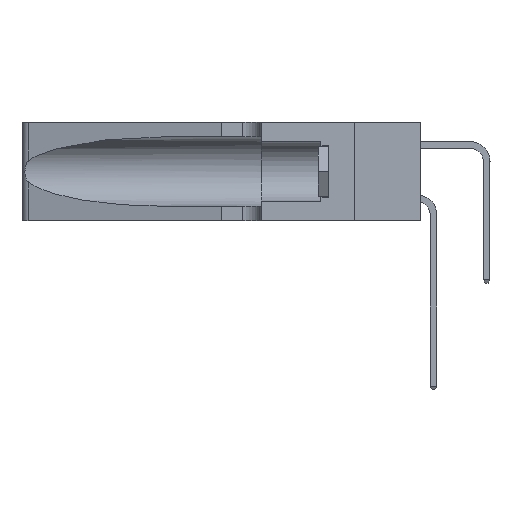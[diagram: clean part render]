
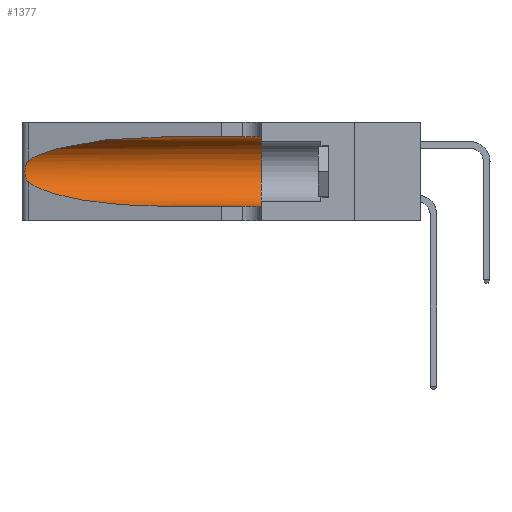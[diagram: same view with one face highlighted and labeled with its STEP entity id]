
A CAD part, left-side view. The second image highlights one B-rep face of the part: STEP entity #1377.
In plain terms, the highlighted cylindrical face has radius 3.308 mm (diameter 6.617 mm), a partial arc.
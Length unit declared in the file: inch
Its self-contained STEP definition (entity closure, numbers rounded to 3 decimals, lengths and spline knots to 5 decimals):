
#92 = ORIENTED_EDGE ( 'NONE', *, *, #10928, .T. ) ;
#417 = CARTESIAN_POINT ( 'NONE',  ( 0.25487, 1.22718, 0.22369 ) ) ;
#531 = CARTESIAN_POINT ( 'NONE',  ( 0.26075, 1.23896, 0.19203 ) ) ;
#1377 = ADVANCED_FACE ( 'NONE', ( #13644 ), #3526, .F. ) ;
#1421 = CARTESIAN_POINT ( 'NONE',  ( 0.1305, 0.72297, 0.05475 ) ) ;
#1494 = CARTESIAN_POINT ( 'NONE',  ( 0.25487, 1.22718, 0.14631 ) ) ;
#2521 = CARTESIAN_POINT ( 'NONE',  ( 0.26017, 1.23833, 0.17102 ) ) ;
#2906 = CARTESIAN_POINT ( 'NONE',  ( 0.1305, 0.35, 0.185 ) ) ;
#3502 = EDGE_CURVE ( 'NONE', #3673, #6131, #13828, .T. ) ;
#3526 = CYLINDRICAL_SURFACE ( 'NONE', #10680, 0.13025 ) ;
#3673 = VERTEX_POINT ( 'NONE', #20260 ) ;
#4228 = VERTEX_POINT ( 'NONE', #1494 ) ;
#4237 =( BOUNDED_CURVE ( )  B_SPLINE_CURVE ( 3, ( #19366, #17523, #21259, #10166 ),
 .UNSPECIFIED., .F., .T. ) 
 B_SPLINE_CURVE_WITH_KNOTS ( ( 4, 4 ),
 ( 3.44316, 4.71239 ),
 .UNSPECIFIED. ) 
 CURVE ( )  GEOMETRIC_REPRESENTATION_ITEM ( )  RATIONAL_B_SPLINE_CURVE ( ( 1., 0.87, 0.87, 1. ) ) 
 REPRESENTATION_ITEM ( '' )  );
#4303 = CARTESIAN_POINT ( 'NONE',  ( 0.1305, 0.72297, 0.31525 ) ) ;
#4442 = CARTESIAN_POINT ( 'NONE',  ( 0.25789, 1.23486, 0.15765 ) ) ;
#4841 = DIRECTION ( 'NONE',  ( 0., 0., 1. ) ) ;
#4911 = EDGE_CURVE ( 'NONE', #12140, #17731, #19085, .T. ) ;
#6131 = VERTEX_POINT ( 'NONE', #20833 ) ;
#6352 = CARTESIAN_POINT ( 'NONE',  ( 0.25555, 1.22994, 0.2215 ) ) ;
#6428 = CARTESIAN_POINT ( 'NONE',  ( 0.25555, 1.22993, 0.14849 ) ) ;
#6671 = CARTESIAN_POINT ( 'NONE',  ( 0.25487, 1.22718, 0.22369 ) ) ;
#7004 = CARTESIAN_POINT ( 'NONE',  ( 0.1305, 1.61858, 0.31525 ) ) ;
#7094 = EDGE_CURVE ( 'NONE', #24322, #6131, #7781, .T. ) ;
#7213 = VECTOR ( 'NONE', #12981, 39.37008 ) ;
#7750 = B_SPLINE_CURVE_WITH_KNOTS ( 'NONE', 3,
 ( #17421, #6352, #21233, #10138, #23103, #12034, #531, #13896, #2521, #15768, #4442, #17578, #6428, #19428 ),
 .UNSPECIFIED., .F., .F.,
 ( 4, 2, 2, 2, 2, 2, 4 ),
 ( 0., 0.00027, 0.00053, 0.00107, 0.0016, 0.00187, 0.00214 ),
 .UNSPECIFIED. ) ;
#7781 = LINE ( 'NONE', #11094, #7213 ) ;
#8578 = CARTESIAN_POINT ( 'NONE',  ( 0.1305, 1.61858, 0.185 ) ) ;
#8790 = ORIENTED_EDGE ( 'NONE', *, *, #20875, .T. ) ;
#8885 = DIRECTION ( 'NONE',  ( 0., -1., 0. ) ) ;
#9174 = DIRECTION ( 'NONE',  ( 0., -1., 0. ) ) ;
#9178 = DIRECTION ( 'NONE',  ( 0., 0., -1. ) ) ;
#9748 = EDGE_LOOP ( 'NONE', ( #18208, #92, #8790, #18884, #14383, #14889 ) ) ;
#10031 = CARTESIAN_POINT ( 'NONE',  ( 0.18966, 0.96281, 0.31525 ) ) ;
#10138 = CARTESIAN_POINT ( 'NONE',  ( 0.25787, 1.23484, 0.2124 ) ) ;
#10166 = CARTESIAN_POINT ( 'NONE',  ( 0.1305, 0.72297, 0.05475 ) ) ;
#10680 = AXIS2_PLACEMENT_3D ( 'NONE', #8578, #9174, #9178 ) ;
#10928 = EDGE_CURVE ( 'NONE', #17731, #4228, #7750, .T. ) ;
#11094 = CARTESIAN_POINT ( 'NONE',  ( 0.1305, 1.61858, 0.05475 ) ) ;
#11936 = CARTESIAN_POINT ( 'NONE',  ( 0.1305, 0.72297, 0.31525 ) ) ;
#12034 = CARTESIAN_POINT ( 'NONE',  ( 0.26018, 1.23835, 0.19895 ) ) ;
#12140 = VERTEX_POINT ( 'NONE', #4303 ) ;
#12981 = DIRECTION ( 'NONE',  ( 0., -1., 0. ) ) ;
#13237 = VECTOR ( 'NONE', #8885, 39.37008 ) ;
#13644 = FACE_OUTER_BOUND ( 'NONE', #9748, .T. ) ;
#13828 = CIRCLE ( 'NONE', #15389, 0.13025 ) ;
#13896 = CARTESIAN_POINT ( 'NONE',  ( 0.26075, 1.23896, 0.178 ) ) ;
#14383 = ORIENTED_EDGE ( 'NONE', *, *, #3502, .F. ) ;
#14889 = ORIENTED_EDGE ( 'NONE', *, *, #22990, .F. ) ;
#15389 = AXIS2_PLACEMENT_3D ( 'NONE', #2906, #16118, #4841 ) ;
#15768 = CARTESIAN_POINT ( 'NONE',  ( 0.25856, 1.23593, 0.16098 ) ) ;
#16118 = DIRECTION ( 'NONE',  ( 0., 1., 0. ) ) ;
#17421 = CARTESIAN_POINT ( 'NONE',  ( 0.25487, 1.22718, 0.22369 ) ) ;
#17523 = CARTESIAN_POINT ( 'NONE',  ( 0.2373, 1.15595, 0.08982 ) ) ;
#17578 = CARTESIAN_POINT ( 'NONE',  ( 0.25639, 1.23186, 0.15144 ) ) ;
#17731 = VERTEX_POINT ( 'NONE', #6671 ) ;
#18208 = ORIENTED_EDGE ( 'NONE', *, *, #4911, .T. ) ;
#18884 = ORIENTED_EDGE ( 'NONE', *, *, #7094, .T. ) ;
#19085 =( BOUNDED_CURVE ( )  B_SPLINE_CURVE ( 3, ( #11936, #10031, #23008, #417 ),
 .UNSPECIFIED., .F., .F. ) 
 B_SPLINE_CURVE_WITH_KNOTS ( ( 4, 4 ),
 ( 1.5708, 2.84003 ),
 .UNSPECIFIED. ) 
 CURVE ( )  GEOMETRIC_REPRESENTATION_ITEM ( )  RATIONAL_B_SPLINE_CURVE ( ( 1., 0.87, 0.87, 1. ) ) 
 REPRESENTATION_ITEM ( '' )  );
#19366 = CARTESIAN_POINT ( 'NONE',  ( 0.25487, 1.22718, 0.14631 ) ) ;
#19428 = CARTESIAN_POINT ( 'NONE',  ( 0.25487, 1.22718, 0.14631 ) ) ;
#20260 = CARTESIAN_POINT ( 'NONE',  ( 0.1305, 0.35, 0.31525 ) ) ;
#20833 = CARTESIAN_POINT ( 'NONE',  ( 0.1305, 0.35, 0.05475 ) ) ;
#20875 = EDGE_CURVE ( 'NONE', #4228, #24322, #4237, .T. ) ;
#21233 = CARTESIAN_POINT ( 'NONE',  ( 0.25639, 1.23184, 0.21858 ) ) ;
#21259 = CARTESIAN_POINT ( 'NONE',  ( 0.18966, 0.96281, 0.05475 ) ) ;
#22990 = EDGE_CURVE ( 'NONE', #12140, #3673, #23052, .T. ) ;
#23008 = CARTESIAN_POINT ( 'NONE',  ( 0.2373, 1.15595, 0.28018 ) ) ;
#23052 = LINE ( 'NONE', #7004, #13237 ) ;
#23103 = CARTESIAN_POINT ( 'NONE',  ( 0.25854, 1.2359, 0.20912 ) ) ;
#24322 = VERTEX_POINT ( 'NONE', #1421 ) ;
